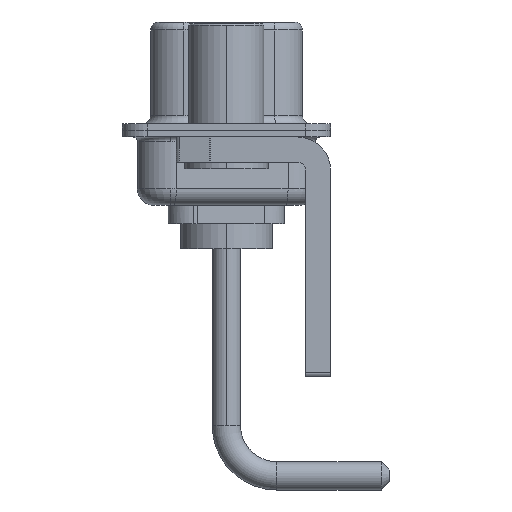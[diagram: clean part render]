
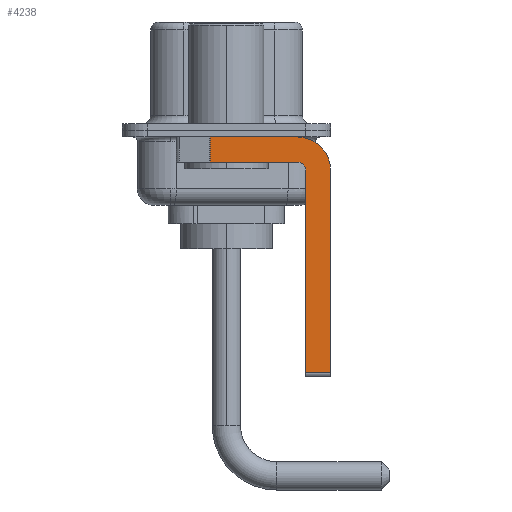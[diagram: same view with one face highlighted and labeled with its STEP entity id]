
A CAD part, left-side view. The second image highlights one B-rep face of the part: STEP entity #4238.
In plain terms, the highlighted planar face has unit normal (-1, 0, 0).
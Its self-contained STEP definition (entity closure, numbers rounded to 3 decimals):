
#63 = ORIENTED_EDGE ( 'NONE', *, *, #2255, .F. ) ;
#71 = VECTOR ( 'NONE', #7995, 1000. ) ;
#324 = VERTEX_POINT ( 'NONE', #5243 ) ;
#754 = VECTOR ( 'NONE', #3371, 1000. ) ;
#913 = DIRECTION ( 'NONE',  ( 0., 0., 1. ) ) ;
#1017 = EDGE_LOOP ( 'NONE', ( #12309, #5647, #7520, #9977, #12068, #7667, #63, #3099 ) ) ;
#1051 = CARTESIAN_POINT ( 'NONE',  ( -2.9, -4.75, -2.4 ) ) ;
#1520 = LINE ( 'NONE', #13137, #71 ) ;
#1619 = EDGE_CURVE ( 'NONE', #324, #2376, #3906, .T. ) ;
#1849 = DIRECTION ( 'NONE',  ( 1., 0., 0. ) ) ;
#1863 = CARTESIAN_POINT ( 'NONE',  ( -2.9, -4.25, -14.55 ) ) ;
#1889 = DIRECTION ( 'NONE',  ( 0., 0., -1. ) ) ;
#1974 = CARTESIAN_POINT ( 'NONE',  ( -2.9, -6.25, -2.4 ) ) ;
#2051 = LINE ( 'NONE', #1974, #3455 ) ;
#2255 = EDGE_CURVE ( 'NONE', #9156, #2645, #2051, .T. ) ;
#2376 = VERTEX_POINT ( 'NONE', #16606 ) ;
#2645 = VERTEX_POINT ( 'NONE', #2983 ) ;
#2705 = DIRECTION ( 'NONE',  ( 0., 0., -1. ) ) ;
#2827 = EDGE_CURVE ( 'NONE', #5025, #16902, #4572, .T. ) ;
#2871 = DIRECTION ( 'NONE',  ( 1., 0., 0. ) ) ;
#2983 = CARTESIAN_POINT ( 'NONE',  ( -2.9, -6.25, -14.55 ) ) ;
#3099 = ORIENTED_EDGE ( 'NONE', *, *, #7936, .F. ) ;
#3371 = DIRECTION ( 'NONE',  ( 0., 1., 0. ) ) ;
#3455 = VECTOR ( 'NONE', #1889, 1000. ) ;
#3495 = AXIS2_PLACEMENT_3D ( 'NONE', #13563, #1849, #7145 ) ;
#3633 = CARTESIAN_POINT ( 'NONE',  ( -2.9, -4.25, -2.4 ) ) ;
#3735 = DIRECTION ( 'NONE',  ( 0., -1., 0. ) ) ;
#3906 = LINE ( 'NONE', #9119, #14546 ) ;
#3925 = EDGE_CURVE ( 'NONE', #16902, #10683, #9561, .T. ) ;
#4238 = ADVANCED_FACE ( 'NONE', ( #13471 ), #5412, .F. ) ;
#4331 = DIRECTION ( 'NONE',  ( 0., -1., 0. ) ) ;
#4487 = VECTOR ( 'NONE', #4331, 1000. ) ;
#4572 = CIRCLE ( 'NONE', #8167, 0.5 ) ;
#5025 = VERTEX_POINT ( 'NONE', #1051 ) ;
#5243 = CARTESIAN_POINT ( 'NONE',  ( -2.9, 0.978, -0.4 ) ) ;
#5412 = PLANE ( 'NONE',  #8907 ) ;
#5486 = CARTESIAN_POINT ( 'NONE',  ( -2.9, -4.75, -14.55 ) ) ;
#5647 = ORIENTED_EDGE ( 'NONE', *, *, #12937, .T. ) ;
#6487 = LINE ( 'NONE', #14455, #14070 ) ;
#7145 = DIRECTION ( 'NONE',  ( 0., 0., -1. ) ) ;
#7229 = DIRECTION ( 'NONE',  ( -1., 0., 0. ) ) ;
#7520 = ORIENTED_EDGE ( 'NONE', *, *, #3925, .F. ) ;
#7667 = ORIENTED_EDGE ( 'NONE', *, *, #16519, .T. ) ;
#7694 = DIRECTION ( 'NONE',  ( 0., 0., 1. ) ) ;
#7936 = EDGE_CURVE ( 'NONE', #2376, #9156, #9239, .T. ) ;
#7995 = DIRECTION ( 'NONE',  ( 0., 0., -1. ) ) ;
#8167 = AXIS2_PLACEMENT_3D ( 'NONE', #3633, #7229, #913 ) ;
#8907 = AXIS2_PLACEMENT_3D ( 'NONE', #13130, #2871, #2705 ) ;
#9119 = CARTESIAN_POINT ( 'NONE',  ( -2.9, 3., -0.4 ) ) ;
#9156 = VERTEX_POINT ( 'NONE', #13170 ) ;
#9239 = CIRCLE ( 'NONE', #3495, 2. ) ;
#9561 = LINE ( 'NONE', #10835, #754 ) ;
#9977 = ORIENTED_EDGE ( 'NONE', *, *, #2827, .F. ) ;
#10683 = VERTEX_POINT ( 'NONE', #14466 ) ;
#10789 = CARTESIAN_POINT ( 'NONE',  ( -2.9, -4.25, -1.9 ) ) ;
#10835 = CARTESIAN_POINT ( 'NONE',  ( -2.9, -4.25, -1.9 ) ) ;
#12068 = ORIENTED_EDGE ( 'NONE', *, *, #16303, .F. ) ;
#12309 = ORIENTED_EDGE ( 'NONE', *, *, #1619, .F. ) ;
#12937 = EDGE_CURVE ( 'NONE', #324, #10683, #1520, .T. ) ;
#13130 = CARTESIAN_POINT ( 'NONE',  ( -2.9, -4.25, -2.4 ) ) ;
#13137 = CARTESIAN_POINT ( 'NONE',  ( -2.9, 0.978, -1.9 ) ) ;
#13170 = CARTESIAN_POINT ( 'NONE',  ( -2.9, -6.25, -2.4 ) ) ;
#13471 = FACE_OUTER_BOUND ( 'NONE', #1017, .T. ) ;
#13563 = CARTESIAN_POINT ( 'NONE',  ( -2.9, -4.25, -2.4 ) ) ;
#14070 = VECTOR ( 'NONE', #7694, 1000. ) ;
#14455 = CARTESIAN_POINT ( 'NONE',  ( -2.9, -4.75, -14.8 ) ) ;
#14466 = CARTESIAN_POINT ( 'NONE',  ( -2.9, 0.978, -1.9 ) ) ;
#14546 = VECTOR ( 'NONE', #3735, 1000. ) ;
#16075 = LINE ( 'NONE', #1863, #4487 ) ;
#16303 = EDGE_CURVE ( 'NONE', #16766, #5025, #6487, .T. ) ;
#16519 = EDGE_CURVE ( 'NONE', #16766, #2645, #16075, .T. ) ;
#16606 = CARTESIAN_POINT ( 'NONE',  ( -2.9, -4.25, -0.4 ) ) ;
#16766 = VERTEX_POINT ( 'NONE', #5486 ) ;
#16902 = VERTEX_POINT ( 'NONE', #10789 ) ;
